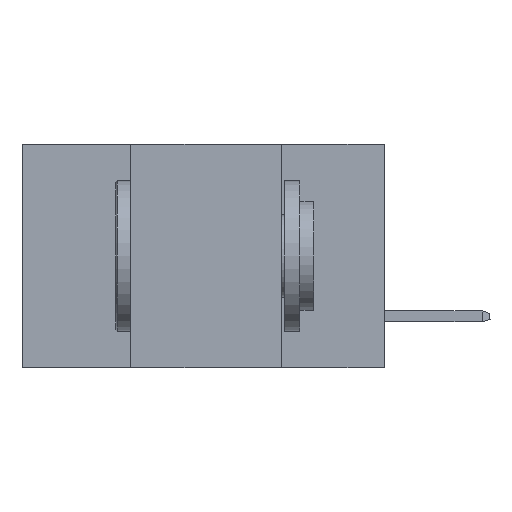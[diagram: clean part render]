
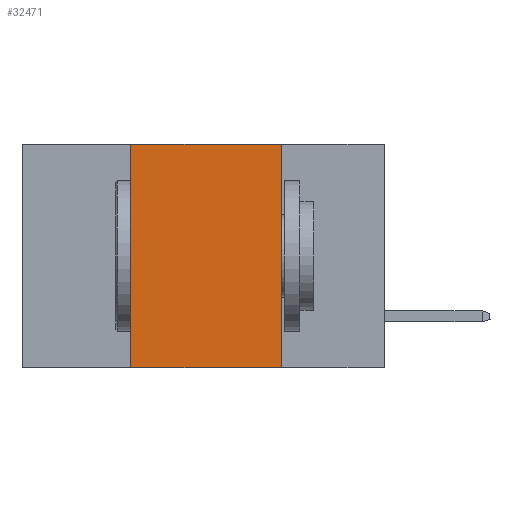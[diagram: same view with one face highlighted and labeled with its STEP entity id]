
A CAD part, left-side view. The second image highlights one B-rep face of the part: STEP entity #32471.
In plain terms, the highlighted planar face has unit normal (-1, 0, 0).
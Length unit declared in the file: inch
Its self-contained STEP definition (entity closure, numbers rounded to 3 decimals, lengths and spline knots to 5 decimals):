
#939 = VERTEX_POINT ( 'NONE', #10520 ) ;
#1558 = DIRECTION ( 'NONE',  ( 0., 0., -1. ) ) ;
#2087 = DIRECTION ( 'NONE',  ( 0., 0., 1. ) ) ;
#2156 = VERTEX_POINT ( 'NONE', #24025 ) ;
#2611 = ORIENTED_EDGE ( 'NONE', *, *, #25374, .F. ) ;
#3964 = EDGE_LOOP ( 'NONE', ( #15740, #2611, #25749, #15896 ) ) ;
#6820 = CARTESIAN_POINT ( 'NONE',  ( 0., 0.6, 0. ) ) ;
#8920 = AXIS2_PLACEMENT_3D ( 'NONE', #6820, #29222, #1558 ) ;
#9967 = CARTESIAN_POINT ( 'NONE',  ( 0., 0.42, -0.37 ) ) ;
#10520 = CARTESIAN_POINT ( 'NONE',  ( 0., 0.42, 0. ) ) ;
#12249 = LINE ( 'NONE', #13359, #24840 ) ;
#13294 = LINE ( 'NONE', #25522, #18021 ) ;
#13359 = CARTESIAN_POINT ( 'NONE',  ( 0., 0.17, 0. ) ) ;
#14806 = VECTOR ( 'NONE', #2087, 39.37008 ) ;
#15740 = ORIENTED_EDGE ( 'NONE', *, *, #17497, .F. ) ;
#15896 = ORIENTED_EDGE ( 'NONE', *, *, #25434, .T. ) ;
#16778 = LINE ( 'NONE', #25956, #18408 ) ;
#17378 = CARTESIAN_POINT ( 'NONE',  ( 0., 0.42, 0. ) ) ;
#17497 = EDGE_CURVE ( 'NONE', #2156, #25499, #12249, .T. ) ;
#18021 = VECTOR ( 'NONE', #22654, 39.37008 ) ;
#18408 = VECTOR ( 'NONE', #23735, 39.37008 ) ;
#21388 = PLANE ( 'NONE',  #8920 ) ;
#22654 = DIRECTION ( 'NONE',  ( 0., -1., 0. ) ) ;
#23735 = DIRECTION ( 'NONE',  ( 0., -1., 0. ) ) ;
#24025 = CARTESIAN_POINT ( 'NONE',  ( 0., 0.17, 0. ) ) ;
#24531 = VERTEX_POINT ( 'NONE', #9967 ) ;
#24840 = VECTOR ( 'NONE', #31018, 39.37008 ) ;
#25374 = EDGE_CURVE ( 'NONE', #939, #2156, #13294, .T. ) ;
#25434 = EDGE_CURVE ( 'NONE', #24531, #25499, #16778, .T. ) ;
#25499 = VERTEX_POINT ( 'NONE', #29288 ) ;
#25522 = CARTESIAN_POINT ( 'NONE',  ( 0., 0.6, 0. ) ) ;
#25749 = ORIENTED_EDGE ( 'NONE', *, *, #31537, .F. ) ;
#25956 = CARTESIAN_POINT ( 'NONE',  ( 0., 0.6, -0.37 ) ) ;
#26228 = LINE ( 'NONE', #17378, #14806 ) ;
#27723 = FACE_OUTER_BOUND ( 'NONE', #3964, .T. ) ;
#29222 = DIRECTION ( 'NONE',  ( 1., 0., 0. ) ) ;
#29288 = CARTESIAN_POINT ( 'NONE',  ( 0., 0.17, -0.37 ) ) ;
#31018 = DIRECTION ( 'NONE',  ( 0., 0., -1. ) ) ;
#31537 = EDGE_CURVE ( 'NONE', #24531, #939, #26228, .T. ) ;
#32471 = ADVANCED_FACE ( 'NONE', ( #27723 ), #21388, .F. ) ;
